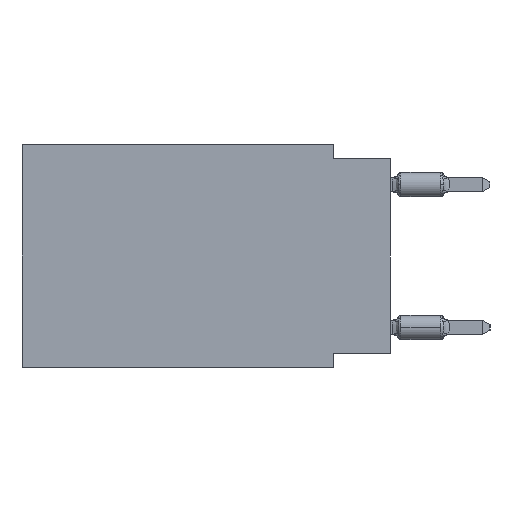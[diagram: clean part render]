
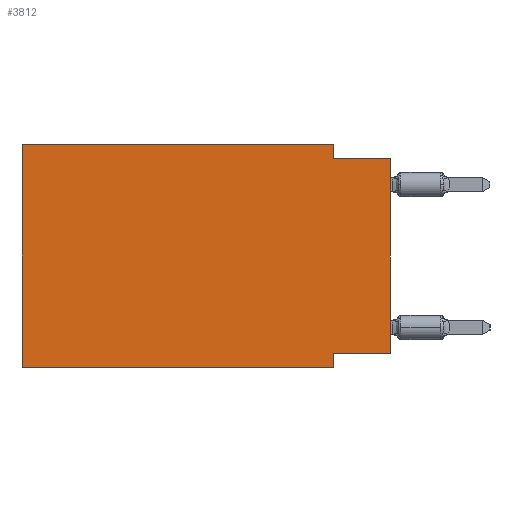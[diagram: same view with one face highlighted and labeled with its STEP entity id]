
A CAD part, left-side view. The second image highlights one B-rep face of the part: STEP entity #3812.
In plain terms, the highlighted planar face has unit normal (-1, 0, 0).
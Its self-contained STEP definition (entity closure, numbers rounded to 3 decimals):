
#759 = LINE ( 'NONE', #38009, #33409 ) ;
#917 = EDGE_CURVE ( 'NONE', #13576, #23257, #9413, .T. ) ;
#1219 = PLANE ( 'NONE',  #25329 ) ;
#2530 = EDGE_CURVE ( 'NONE', #20148, #5930, #4399, .T. ) ;
#3104 = DIRECTION ( 'NONE',  ( 0., -1., 0. ) ) ;
#3812 = ADVANCED_FACE ( 'NONE', ( #49566 ), #1219, .F. ) ;
#3989 = ORIENTED_EDGE ( 'NONE', *, *, #42841, .F. ) ;
#4399 = LINE ( 'NONE', #20504, #33798 ) ;
#4493 = CARTESIAN_POINT ( 'NONE',  ( 0., 16.383, -9.906 ) ) ;
#5523 = VERTEX_POINT ( 'NONE', #32167 ) ;
#5716 = ORIENTED_EDGE ( 'NONE', *, *, #51233, .F. ) ;
#5866 = EDGE_CURVE ( 'NONE', #5523, #20148, #45911, .T. ) ;
#5930 = VERTEX_POINT ( 'NONE', #27102 ) ;
#7110 = VECTOR ( 'NONE', #3104, 1000. ) ;
#7762 = LINE ( 'NONE', #19387, #7864 ) ;
#7864 = VECTOR ( 'NONE', #43421, 1000. ) ;
#8382 = EDGE_CURVE ( 'NONE', #5930, #23257, #35072, .T. ) ;
#9413 = LINE ( 'NONE', #49035, #37115 ) ;
#10982 = CARTESIAN_POINT ( 'NONE',  ( 0., 0., -0.635 ) ) ;
#11592 = EDGE_CURVE ( 'NONE', #44649, #5523, #759, .T. ) ;
#13203 = DIRECTION ( 'NONE',  ( 0., -1., 0. ) ) ;
#13230 = VERTEX_POINT ( 'NONE', #21305 ) ;
#13576 = VERTEX_POINT ( 'NONE', #44163 ) ;
#13646 = CARTESIAN_POINT ( 'NONE',  ( 0., 16.383, 0. ) ) ;
#14445 = ORIENTED_EDGE ( 'NONE', *, *, #21363, .T. ) ;
#15579 = ORIENTED_EDGE ( 'NONE', *, *, #5866, .F. ) ;
#16405 = ORIENTED_EDGE ( 'NONE', *, *, #917, .T. ) ;
#16804 = DIRECTION ( 'NONE',  ( 0., 0., -1. ) ) ;
#17346 = DIRECTION ( 'NONE',  ( 1., 0., 0. ) ) ;
#17908 = CARTESIAN_POINT ( 'NONE',  ( 0., 16.383, 0. ) ) ;
#17912 = VECTOR ( 'NONE', #34021, 1000. ) ;
#18150 = CARTESIAN_POINT ( 'NONE',  ( 0., 2.54, -9.906 ) ) ;
#19387 = CARTESIAN_POINT ( 'NONE',  ( 0., 2.54, -9.906 ) ) ;
#19529 = ORIENTED_EDGE ( 'NONE', *, *, #8382, .F. ) ;
#20148 = VERTEX_POINT ( 'NONE', #50853 ) ;
#20504 = CARTESIAN_POINT ( 'NONE',  ( 0., 2.54, 0. ) ) ;
#20612 = VECTOR ( 'NONE', #22943, 1000. ) ;
#21305 = CARTESIAN_POINT ( 'NONE',  ( 0., 2.54, -9.271 ) ) ;
#21363 = EDGE_CURVE ( 'NONE', #44649, #23120, #40685, .T. ) ;
#21547 = DIRECTION ( 'NONE',  ( 0., 0., -1. ) ) ;
#22943 = DIRECTION ( 'NONE',  ( 0., 1., 0. ) ) ;
#23120 = VERTEX_POINT ( 'NONE', #18150 ) ;
#23257 = VERTEX_POINT ( 'NONE', #10982 ) ;
#25329 = AXIS2_PLACEMENT_3D ( 'NONE', #13646, #17346, #16804 ) ;
#27102 = CARTESIAN_POINT ( 'NONE',  ( 0., 2.54, -0.635 ) ) ;
#29548 = DIRECTION ( 'NONE',  ( 0., 0., 1. ) ) ;
#31094 = CARTESIAN_POINT ( 'NONE',  ( 0., 0., -0.635 ) ) ;
#32167 = CARTESIAN_POINT ( 'NONE',  ( 0., 16.383, 0. ) ) ;
#33409 = VECTOR ( 'NONE', #29548, 1000. ) ;
#33798 = VECTOR ( 'NONE', #21547, 1000. ) ;
#34021 = DIRECTION ( 'NONE',  ( 0., -1., 0. ) ) ;
#34591 = LINE ( 'NONE', #50695, #20612 ) ;
#35072 = LINE ( 'NONE', #31094, #7110 ) ;
#36363 = CARTESIAN_POINT ( 'NONE',  ( 0., 16.383, -9.906 ) ) ;
#36887 = DIRECTION ( 'NONE',  ( 0., 0., 1. ) ) ;
#37115 = VECTOR ( 'NONE', #36887, 1000. ) ;
#38009 = CARTESIAN_POINT ( 'NONE',  ( 0., 16.383, 0. ) ) ;
#39354 = ORIENTED_EDGE ( 'NONE', *, *, #2530, .F. ) ;
#40685 = LINE ( 'NONE', #4493, #41930 ) ;
#41930 = VECTOR ( 'NONE', #13203, 1000. ) ;
#42841 = EDGE_CURVE ( 'NONE', #13576, #13230, #34591, .T. ) ;
#43421 = DIRECTION ( 'NONE',  ( 0., 0., -1. ) ) ;
#44163 = CARTESIAN_POINT ( 'NONE',  ( 0., 0., -9.271 ) ) ;
#44649 = VERTEX_POINT ( 'NONE', #36363 ) ;
#45911 = LINE ( 'NONE', #17908, #17912 ) ;
#46128 = EDGE_LOOP ( 'NONE', ( #16405, #19529, #39354, #15579, #51661, #14445, #5716, #3989 ) ) ;
#49035 = CARTESIAN_POINT ( 'NONE',  ( 0., 0., 0. ) ) ;
#49566 = FACE_OUTER_BOUND ( 'NONE', #46128, .T. ) ;
#50695 = CARTESIAN_POINT ( 'NONE',  ( 0., 0., -9.271 ) ) ;
#50853 = CARTESIAN_POINT ( 'NONE',  ( 0., 2.54, 0. ) ) ;
#51233 = EDGE_CURVE ( 'NONE', #13230, #23120, #7762, .T. ) ;
#51661 = ORIENTED_EDGE ( 'NONE', *, *, #11592, .F. ) ;
